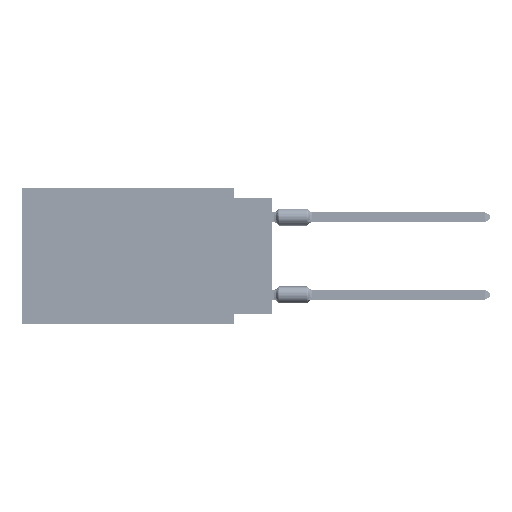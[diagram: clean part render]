
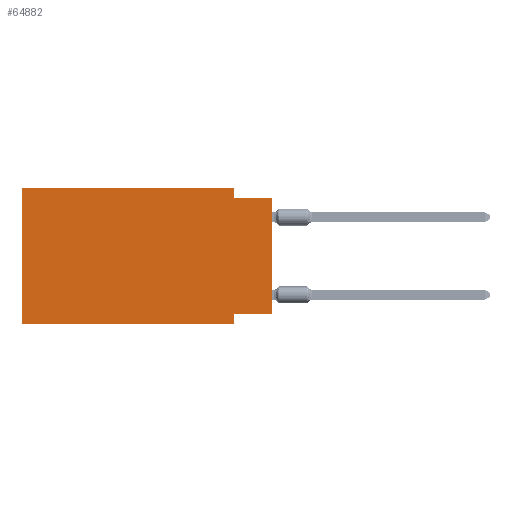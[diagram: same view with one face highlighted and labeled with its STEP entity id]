
A CAD part, left-side view. The second image highlights one B-rep face of the part: STEP entity #64882.
In plain terms, the highlighted planar face has unit normal (-1, 0, 0).
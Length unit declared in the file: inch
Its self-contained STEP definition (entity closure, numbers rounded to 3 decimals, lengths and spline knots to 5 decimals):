
#104 = EDGE_CURVE ( 'NONE', #29755, #49167, #20097, .T. ) ;
#1210 = ORIENTED_EDGE ( 'NONE', *, *, #3827, .T. ) ;
#1422 = ORIENTED_EDGE ( 'NONE', *, *, #43527, .F. ) ;
#3087 = EDGE_CURVE ( 'NONE', #43132, #24026, #61311, .T. ) ;
#3676 = DIRECTION ( 'NONE',  ( 0., -1., 0. ) ) ;
#3827 = EDGE_CURVE ( 'NONE', #3899, #24026, #45366, .T. ) ;
#3899 = VERTEX_POINT ( 'NONE', #60706 ) ;
#4513 = DIRECTION ( 'NONE',  ( 0., 0., -1. ) ) ;
#4652 = CARTESIAN_POINT ( 'NONE',  ( 0., 0.645, 0. ) ) ;
#5090 = ORIENTED_EDGE ( 'NONE', *, *, #18015, .T. ) ;
#5673 = VECTOR ( 'NONE', #3676, 39.37008 ) ;
#6079 = CARTESIAN_POINT ( 'NONE',  ( 0., 0.1, 0. ) ) ;
#10724 = LINE ( 'NONE', #4652, #56268 ) ;
#12457 = CARTESIAN_POINT ( 'NONE',  ( 0., 0., -0.325 ) ) ;
#13412 = VECTOR ( 'NONE', #27763, 39.37008 ) ;
#15698 = EDGE_LOOP ( 'NONE', ( #5090, #69705, #68420, #71536, #1422, #1210, #70928, #47611 ) ) ;
#15787 = VECTOR ( 'NONE', #17192, 39.37008 ) ;
#16456 = VECTOR ( 'NONE', #37107, 39.37008 ) ;
#17192 = DIRECTION ( 'NONE',  ( 0., 0., -1. ) ) ;
#18015 = EDGE_CURVE ( 'NONE', #54548, #49167, #75507, .T. ) ;
#18031 = FACE_OUTER_BOUND ( 'NONE', #15698, .T. ) ;
#20097 = LINE ( 'NONE', #69491, #13412 ) ;
#23072 = VECTOR ( 'NONE', #44031, 39.37008 ) ;
#23914 = CARTESIAN_POINT ( 'NONE',  ( 0., 0.1, 0. ) ) ;
#24026 = VERTEX_POINT ( 'NONE', #64300 ) ;
#27763 = DIRECTION ( 'NONE',  ( 0., -1., 0. ) ) ;
#29755 = VERTEX_POINT ( 'NONE', #52320 ) ;
#32424 = EDGE_CURVE ( 'NONE', #55035, #75697, #10724, .T. ) ;
#36701 = EDGE_CURVE ( 'NONE', #75697, #29755, #67231, .T. ) ;
#37107 = DIRECTION ( 'NONE',  ( 0., 1., 0. ) ) ;
#39395 = AXIS2_PLACEMENT_3D ( 'NONE', #73482, #73891, #62140 ) ;
#40600 = CARTESIAN_POINT ( 'NONE',  ( 0., 0., -0.325 ) ) ;
#43132 = VERTEX_POINT ( 'NONE', #56284 ) ;
#43527 = EDGE_CURVE ( 'NONE', #3899, #55035, #50518, .T. ) ;
#43902 = PLANE ( 'NONE',  #39395 ) ;
#44031 = DIRECTION ( 'NONE',  ( 0., 0., 1. ) ) ;
#44333 = DIRECTION ( 'NONE',  ( 0., 0., 1. ) ) ;
#45366 = LINE ( 'NONE', #70076, #5673 ) ;
#47611 = ORIENTED_EDGE ( 'NONE', *, *, #50359, .F. ) ;
#49167 = VERTEX_POINT ( 'NONE', #53759 ) ;
#50359 = EDGE_CURVE ( 'NONE', #54548, #43132, #67514, .T. ) ;
#50518 = LINE ( 'NONE', #75210, #23072 ) ;
#52320 = CARTESIAN_POINT ( 'NONE',  ( 0., 0.1, -0.025 ) ) ;
#53759 = CARTESIAN_POINT ( 'NONE',  ( 0., 0., -0.025 ) ) ;
#54548 = VERTEX_POINT ( 'NONE', #40600 ) ;
#55035 = VERTEX_POINT ( 'NONE', #77354 ) ;
#55237 = CARTESIAN_POINT ( 'NONE',  ( 0., 0.1, -0.35 ) ) ;
#56268 = VECTOR ( 'NONE', #66961, 39.37008 ) ;
#56284 = CARTESIAN_POINT ( 'NONE',  ( 0., 0.1, -0.325 ) ) ;
#59539 = VECTOR ( 'NONE', #44333, 39.37008 ) ;
#60706 = CARTESIAN_POINT ( 'NONE',  ( 0., 0.645, -0.35 ) ) ;
#61311 = LINE ( 'NONE', #55237, #15787 ) ;
#62140 = DIRECTION ( 'NONE',  ( 0., 0., -1. ) ) ;
#62563 = CARTESIAN_POINT ( 'NONE',  ( 0., 0., 0. ) ) ;
#64300 = CARTESIAN_POINT ( 'NONE',  ( 0., 0.1, -0.35 ) ) ;
#64882 = ADVANCED_FACE ( 'NONE', ( #18031 ), #43902, .F. ) ;
#66961 = DIRECTION ( 'NONE',  ( 0., -1., 0. ) ) ;
#67231 = LINE ( 'NONE', #23914, #67779 ) ;
#67514 = LINE ( 'NONE', #12457, #16456 ) ;
#67779 = VECTOR ( 'NONE', #4513, 39.37008 ) ;
#68420 = ORIENTED_EDGE ( 'NONE', *, *, #36701, .F. ) ;
#69491 = CARTESIAN_POINT ( 'NONE',  ( 0., 0., -0.025 ) ) ;
#69705 = ORIENTED_EDGE ( 'NONE', *, *, #104, .F. ) ;
#70076 = CARTESIAN_POINT ( 'NONE',  ( 0., 0.645, -0.35 ) ) ;
#70928 = ORIENTED_EDGE ( 'NONE', *, *, #3087, .F. ) ;
#71536 = ORIENTED_EDGE ( 'NONE', *, *, #32424, .F. ) ;
#73482 = CARTESIAN_POINT ( 'NONE',  ( 0., 0.645, 0. ) ) ;
#73891 = DIRECTION ( 'NONE',  ( 1., 0., 0. ) ) ;
#75210 = CARTESIAN_POINT ( 'NONE',  ( 0., 0.645, 0. ) ) ;
#75507 = LINE ( 'NONE', #62563, #59539 ) ;
#75697 = VERTEX_POINT ( 'NONE', #6079 ) ;
#77354 = CARTESIAN_POINT ( 'NONE',  ( 0., 0.645, 0. ) ) ;
